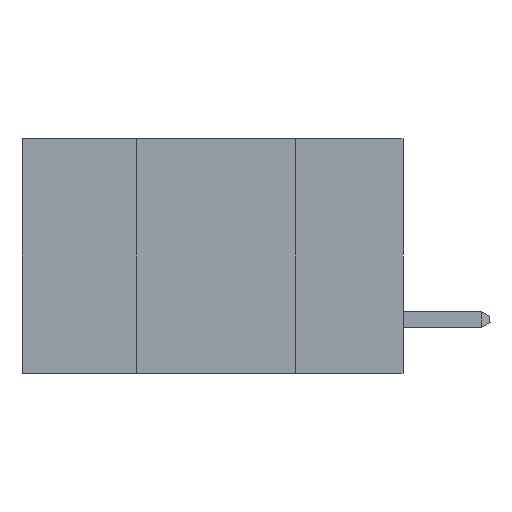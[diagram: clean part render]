
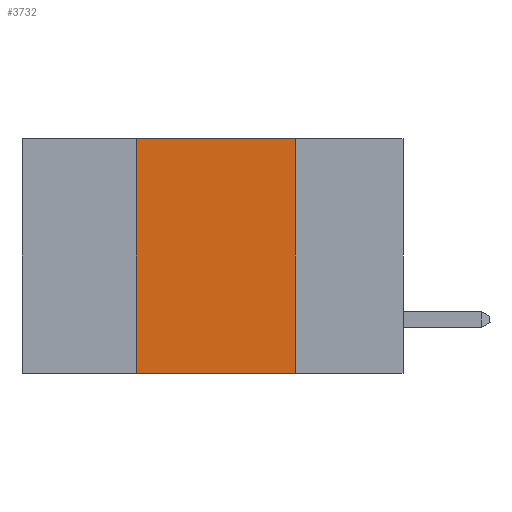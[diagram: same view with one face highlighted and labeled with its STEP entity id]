
A CAD part, left-side view. The second image highlights one B-rep face of the part: STEP entity #3732.
In plain terms, the highlighted planar face has unit normal (-1, 0, 0).
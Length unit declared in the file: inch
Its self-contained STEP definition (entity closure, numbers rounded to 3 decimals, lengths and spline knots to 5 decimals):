
#121 = EDGE_CURVE ( 'NONE', #12570, #14990, #9723, .T. ) ;
#214 = EDGE_CURVE ( 'NONE', #2397, #14990, #10476, .T. ) ;
#410 = CARTESIAN_POINT ( 'NONE',  ( 0., 0.6, 0. ) ) ;
#829 = VECTOR ( 'NONE', #7183, 39.37008 ) ;
#1168 = CARTESIAN_POINT ( 'NONE',  ( 0., 0.17, 0. ) ) ;
#1339 = VECTOR ( 'NONE', #12303, 39.37008 ) ;
#1351 = ORIENTED_EDGE ( 'NONE', *, *, #11307, .F. ) ;
#1625 = CARTESIAN_POINT ( 'NONE',  ( 0., 0.42, -0.37 ) ) ;
#1826 = CARTESIAN_POINT ( 'NONE',  ( 0., 0.42, 0. ) ) ;
#2020 = VERTEX_POINT ( 'NONE', #1826 ) ;
#2081 = FACE_OUTER_BOUND ( 'NONE', #3130, .T. ) ;
#2232 = AXIS2_PLACEMENT_3D ( 'NONE', #410, #8852, #6486 ) ;
#2397 = VERTEX_POINT ( 'NONE', #1625 ) ;
#3130 = EDGE_LOOP ( 'NONE', ( #10928, #1351, #6443, #7628 ) ) ;
#3732 = ADVANCED_FACE ( 'NONE', ( #2081 ), #14903, .F. ) ;
#3799 = EDGE_CURVE ( 'NONE', #2397, #2020, #12429, .T. ) ;
#5303 = LINE ( 'NONE', #14690, #1339 ) ;
#5934 = VECTOR ( 'NONE', #14241, 39.37008 ) ;
#6443 = ORIENTED_EDGE ( 'NONE', *, *, #3799, .F. ) ;
#6486 = DIRECTION ( 'NONE',  ( 0., 0., -1. ) ) ;
#6583 = CARTESIAN_POINT ( 'NONE',  ( 0., 0.42, 0. ) ) ;
#7183 = DIRECTION ( 'NONE',  ( 0., -1., 0. ) ) ;
#7313 = CARTESIAN_POINT ( 'NONE',  ( 0., 0.17, -0.37 ) ) ;
#7628 = ORIENTED_EDGE ( 'NONE', *, *, #214, .T. ) ;
#8086 = VECTOR ( 'NONE', #15103, 39.37008 ) ;
#8264 = CARTESIAN_POINT ( 'NONE',  ( 0., 0.17, 0. ) ) ;
#8342 = CARTESIAN_POINT ( 'NONE',  ( 0., 0.6, -0.37 ) ) ;
#8852 = DIRECTION ( 'NONE',  ( 1., 0., 0. ) ) ;
#9723 = LINE ( 'NONE', #8264, #5934 ) ;
#10476 = LINE ( 'NONE', #8342, #829 ) ;
#10928 = ORIENTED_EDGE ( 'NONE', *, *, #121, .F. ) ;
#11307 = EDGE_CURVE ( 'NONE', #2020, #12570, #5303, .T. ) ;
#12303 = DIRECTION ( 'NONE',  ( 0., -1., 0. ) ) ;
#12429 = LINE ( 'NONE', #6583, #8086 ) ;
#12570 = VERTEX_POINT ( 'NONE', #1168 ) ;
#14241 = DIRECTION ( 'NONE',  ( 0., 0., -1. ) ) ;
#14690 = CARTESIAN_POINT ( 'NONE',  ( 0., 0.6, 0. ) ) ;
#14903 = PLANE ( 'NONE',  #2232 ) ;
#14990 = VERTEX_POINT ( 'NONE', #7313 ) ;
#15103 = DIRECTION ( 'NONE',  ( 0., 0., 1. ) ) ;
